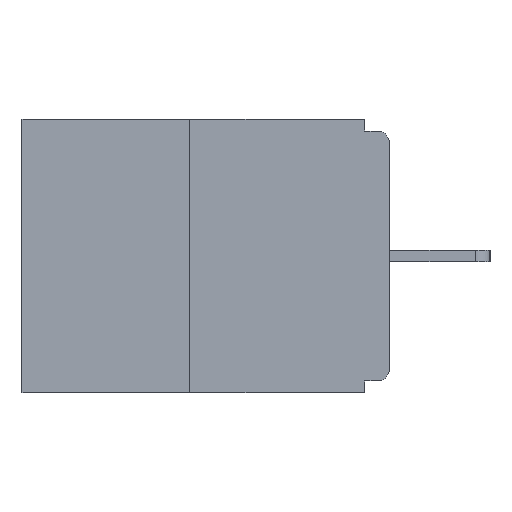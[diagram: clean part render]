
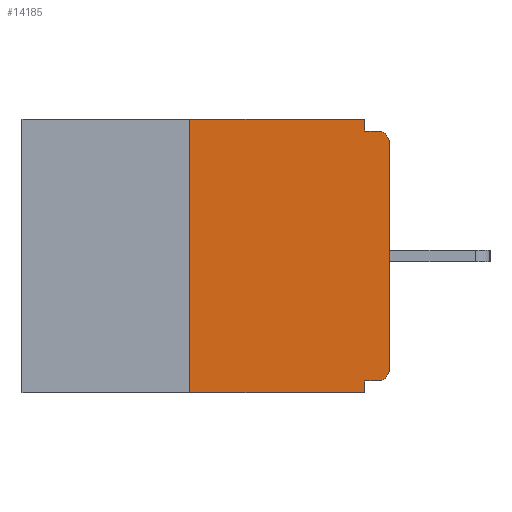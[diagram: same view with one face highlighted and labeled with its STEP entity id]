
A CAD part, left-side view. The second image highlights one B-rep face of the part: STEP entity #14185.
In plain terms, the highlighted planar face has unit normal (-1, 0, 0).
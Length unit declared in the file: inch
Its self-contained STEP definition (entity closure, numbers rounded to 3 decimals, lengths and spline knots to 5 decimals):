
#533 = ORIENTED_EDGE ( 'NONE', *, *, #4264, .T. ) ;
#1162 = EDGE_CURVE ( 'NONE', #7608, #7327, #13536, .T. ) ;
#1294 = VERTEX_POINT ( 'NONE', #7216 ) ;
#1466 = VECTOR ( 'NONE', #9856, 39.37008 ) ;
#1536 = CARTESIAN_POINT ( 'NONE',  ( 0., 0.25, -0.343 ) ) ;
#1614 = LINE ( 'NONE', #1904, #12112 ) ;
#1625 = EDGE_CURVE ( 'NONE', #17806, #10767, #5911, .T. ) ;
#1754 = ORIENTED_EDGE ( 'NONE', *, *, #1906, .F. ) ;
#1904 = CARTESIAN_POINT ( 'NONE',  ( 0., 0., -0.015 ) ) ;
#1906 = EDGE_CURVE ( 'NONE', #10767, #3985, #10754, .T. ) ;
#2108 = CARTESIAN_POINT ( 'NONE',  ( 0., 0., -0.328 ) ) ;
#2287 = ORIENTED_EDGE ( 'NONE', *, *, #1625, .F. ) ;
#2639 = CARTESIAN_POINT ( 'NONE',  ( 0., 0., 0. ) ) ;
#2643 = EDGE_CURVE ( 'NONE', #7608, #3985, #4588, .T. ) ;
#2680 = ORIENTED_EDGE ( 'NONE', *, *, #6824, .T. ) ;
#3668 = VERTEX_POINT ( 'NONE', #16007 ) ;
#3759 = EDGE_CURVE ( 'NONE', #14299, #3668, #6891, .T. ) ;
#3985 = VERTEX_POINT ( 'NONE', #11833 ) ;
#3990 = DIRECTION ( 'NONE',  ( 0., 0., -1. ) ) ;
#4051 = VECTOR ( 'NONE', #14141, 39.37008 ) ;
#4264 = EDGE_CURVE ( 'NONE', #3668, #5094, #6687, .T. ) ;
#4588 = LINE ( 'NONE', #4676, #11545 ) ;
#4594 = CARTESIAN_POINT ( 'NONE',  ( 0., 0.015, -0.328 ) ) ;
#4649 = CARTESIAN_POINT ( 'NONE',  ( 0., 0.46, 0. ) ) ;
#4676 = CARTESIAN_POINT ( 'NONE',  ( 0., 0.46, -0.343 ) ) ;
#5094 = VERTEX_POINT ( 'NONE', #15817 ) ;
#5911 = LINE ( 'NONE', #2108, #9293 ) ;
#6059 = DIRECTION ( 'NONE',  ( 0., -1., 0. ) ) ;
#6414 = FACE_OUTER_BOUND ( 'NONE', #10821, .T. ) ;
#6495 = DIRECTION ( 'NONE',  ( 0., 0., -1. ) ) ;
#6687 = CIRCLE ( 'NONE', #13305, 0.015 ) ;
#6824 = EDGE_CURVE ( 'NONE', #17806, #14299, #7575, .T. ) ;
#6891 = LINE ( 'NONE', #2639, #1466 ) ;
#7028 = ORIENTED_EDGE ( 'NONE', *, *, #16860, .F. ) ;
#7216 = CARTESIAN_POINT ( 'NONE',  ( 0., 0.031, -0.015 ) ) ;
#7281 = LINE ( 'NONE', #4649, #4051 ) ;
#7327 = VERTEX_POINT ( 'NONE', #8232 ) ;
#7361 = DIRECTION ( 'NONE',  ( 0., 0., -1. ) ) ;
#7575 = CIRCLE ( 'NONE', #11325, 0.015 ) ;
#7593 = PLANE ( 'NONE',  #17726 ) ;
#7608 = VERTEX_POINT ( 'NONE', #1536 ) ;
#8172 = CARTESIAN_POINT ( 'NONE',  ( 0., 0.031, 0. ) ) ;
#8212 = ORIENTED_EDGE ( 'NONE', *, *, #3759, .T. ) ;
#8232 = CARTESIAN_POINT ( 'NONE',  ( 0., 0.25, 0. ) ) ;
#8389 = DIRECTION ( 'NONE',  ( 0., 0., 1. ) ) ;
#8620 = LINE ( 'NONE', #8798, #16315 ) ;
#8798 = CARTESIAN_POINT ( 'NONE',  ( 0., 0.031, 0. ) ) ;
#9280 = DIRECTION ( 'NONE',  ( -1., 0., 0. ) ) ;
#9293 = VECTOR ( 'NONE', #11413, 39.37008 ) ;
#9856 = DIRECTION ( 'NONE',  ( 0., 0., 1. ) ) ;
#10100 = DIRECTION ( 'NONE',  ( 0., -1., 0. ) ) ;
#10133 = CARTESIAN_POINT ( 'NONE',  ( 0., 0.031, -0.328 ) ) ;
#10634 = CARTESIAN_POINT ( 'NONE',  ( 0., 0.46, 0. ) ) ;
#10754 = LINE ( 'NONE', #16366, #15983 ) ;
#10767 = VERTEX_POINT ( 'NONE', #10133 ) ;
#10821 = EDGE_LOOP ( 'NONE', ( #16139, #17651, #12871, #1754, #2287, #2680, #8212, #533, #15847, #7028 ) ) ;
#11090 = CARTESIAN_POINT ( 'NONE',  ( 0., 0.25, 0. ) ) ;
#11167 = EDGE_CURVE ( 'NONE', #1294, #5094, #1614, .T. ) ;
#11325 = AXIS2_PLACEMENT_3D ( 'NONE', #14390, #9280, #6495 ) ;
#11413 = DIRECTION ( 'NONE',  ( 0., 1., 0. ) ) ;
#11545 = VECTOR ( 'NONE', #10100, 39.37008 ) ;
#11576 = VECTOR ( 'NONE', #8389, 39.37008 ) ;
#11833 = CARTESIAN_POINT ( 'NONE',  ( 0., 0.031, -0.343 ) ) ;
#11851 = EDGE_CURVE ( 'NONE', #7327, #15536, #7281, .T. ) ;
#12112 = VECTOR ( 'NONE', #6059, 39.37008 ) ;
#12459 = CARTESIAN_POINT ( 'NONE',  ( 0., 0.015, -0.03 ) ) ;
#12871 = ORIENTED_EDGE ( 'NONE', *, *, #2643, .T. ) ;
#13305 = AXIS2_PLACEMENT_3D ( 'NONE', #12459, #15432, #15615 ) ;
#13536 = LINE ( 'NONE', #11090, #11576 ) ;
#14141 = DIRECTION ( 'NONE',  ( 0., -1., 0. ) ) ;
#14185 = ADVANCED_FACE ( 'NONE', ( #6414 ), #7593, .F. ) ;
#14299 = VERTEX_POINT ( 'NONE', #17788 ) ;
#14390 = CARTESIAN_POINT ( 'NONE',  ( 0., 0.015, -0.313 ) ) ;
#14798 = DIRECTION ( 'NONE',  ( 0., 0., -1. ) ) ;
#15432 = DIRECTION ( 'NONE',  ( -1., 0., 0. ) ) ;
#15536 = VERTEX_POINT ( 'NONE', #8172 ) ;
#15615 = DIRECTION ( 'NONE',  ( 0., 0., -1. ) ) ;
#15817 = CARTESIAN_POINT ( 'NONE',  ( 0., 0.015, -0.015 ) ) ;
#15847 = ORIENTED_EDGE ( 'NONE', *, *, #11167, .F. ) ;
#15983 = VECTOR ( 'NONE', #3990, 39.37008 ) ;
#16007 = CARTESIAN_POINT ( 'NONE',  ( 0., 0., -0.03 ) ) ;
#16139 = ORIENTED_EDGE ( 'NONE', *, *, #11851, .F. ) ;
#16315 = VECTOR ( 'NONE', #7361, 39.37008 ) ;
#16366 = CARTESIAN_POINT ( 'NONE',  ( 0., 0.031, -0.343 ) ) ;
#16860 = EDGE_CURVE ( 'NONE', #15536, #1294, #8620, .T. ) ;
#17347 = DIRECTION ( 'NONE',  ( 1., 0., 0. ) ) ;
#17651 = ORIENTED_EDGE ( 'NONE', *, *, #1162, .F. ) ;
#17726 = AXIS2_PLACEMENT_3D ( 'NONE', #10634, #17347, #14798 ) ;
#17788 = CARTESIAN_POINT ( 'NONE',  ( 0., 0., -0.313 ) ) ;
#17806 = VERTEX_POINT ( 'NONE', #4594 ) ;
